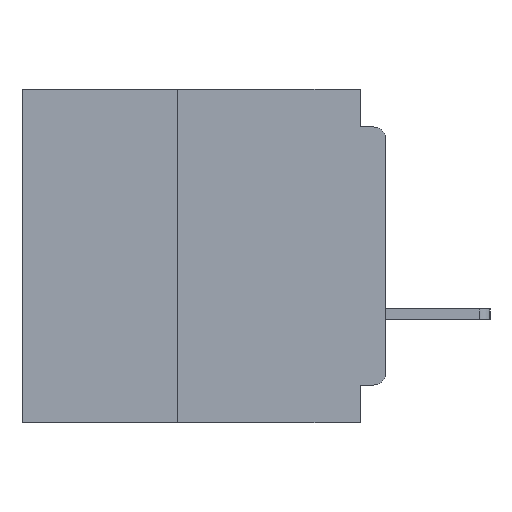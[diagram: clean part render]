
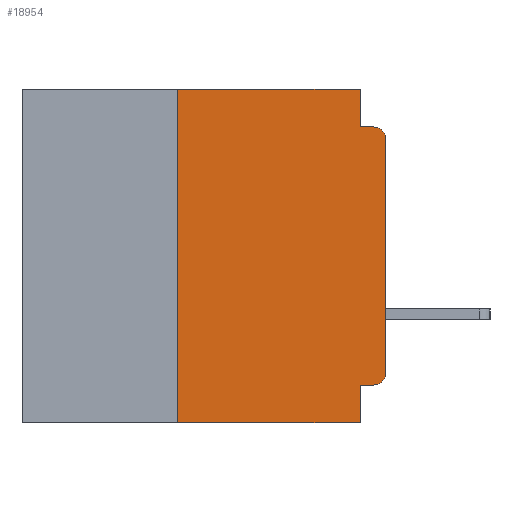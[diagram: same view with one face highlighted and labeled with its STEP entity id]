
A CAD part, left-side view. The second image highlights one B-rep face of the part: STEP entity #18954.
In plain terms, the highlighted planar face has unit normal (-1, 0, 0).
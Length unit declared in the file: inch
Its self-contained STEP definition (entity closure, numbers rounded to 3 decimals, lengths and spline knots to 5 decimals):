
#171 = EDGE_CURVE ( 'NONE', #24184, #37073, #20855, .T. ) ;
#1315 = EDGE_CURVE ( 'NONE', #27037, #25152, #16769, .T. ) ;
#1594 = VERTEX_POINT ( 'NONE', #29103 ) ;
#2092 = DIRECTION ( 'NONE',  ( 0., 0., -1. ) ) ;
#2588 = VECTOR ( 'NONE', #40106, 39.37008 ) ;
#3634 = PLANE ( 'NONE',  #33604 ) ;
#4364 = LINE ( 'NONE', #22673, #41997 ) ;
#5038 = ORIENTED_EDGE ( 'NONE', *, *, #36987, .T. ) ;
#8489 = VERTEX_POINT ( 'NONE', #29799 ) ;
#8672 = DIRECTION ( 'NONE',  ( 0., 1., 0. ) ) ;
#10243 = ORIENTED_EDGE ( 'NONE', *, *, #1315, .T. ) ;
#10694 = CARTESIAN_POINT ( 'NONE',  ( 0., 0.437, -0.4 ) ) ;
#10991 = DIRECTION ( 'NONE',  ( 1., 0., 0. ) ) ;
#11439 = CARTESIAN_POINT ( 'NONE',  ( 0., 0.031, -0.4 ) ) ;
#11780 = LINE ( 'NONE', #34227, #41982 ) ;
#11825 = DIRECTION ( 'NONE',  ( 0., -1., 0. ) ) ;
#12669 = EDGE_CURVE ( 'NONE', #1594, #23631, #24501, .T. ) ;
#12686 = ORIENTED_EDGE ( 'NONE', *, *, #22652, .F. ) ;
#12821 = CARTESIAN_POINT ( 'NONE',  ( 0., 0.25, -0.4 ) ) ;
#12879 = CARTESIAN_POINT ( 'NONE',  ( 0., 0.015, -0.045 ) ) ;
#13369 = DIRECTION ( 'NONE',  ( 0., 0., -1. ) ) ;
#13486 = CARTESIAN_POINT ( 'NONE',  ( 0., 0.015, -0.355 ) ) ;
#13913 = DIRECTION ( 'NONE',  ( -1., 0., 0. ) ) ;
#14073 = CARTESIAN_POINT ( 'NONE',  ( 0., 0.015, -0.34 ) ) ;
#14104 = EDGE_LOOP ( 'NONE', ( #5038, #17039, #27082, #12686, #37196, #30086, #36721, #33776, #36097, #10243 ) ) ;
#14174 = CARTESIAN_POINT ( 'NONE',  ( 0., 0., -0.045 ) ) ;
#14814 = CARTESIAN_POINT ( 'NONE',  ( 0., 0., -0.34 ) ) ;
#14836 = VECTOR ( 'NONE', #32329, 39.37008 ) ;
#15529 = CARTESIAN_POINT ( 'NONE',  ( 0., 0.015, -0.06 ) ) ;
#16284 = CARTESIAN_POINT ( 'NONE',  ( 0., 0., -0.06 ) ) ;
#16769 = CIRCLE ( 'NONE', #42944, 0.015 ) ;
#16864 = VERTEX_POINT ( 'NONE', #17652 ) ;
#17039 = ORIENTED_EDGE ( 'NONE', *, *, #42657, .T. ) ;
#17652 = CARTESIAN_POINT ( 'NONE',  ( 0., 0.25, 0. ) ) ;
#18551 = VECTOR ( 'NONE', #2092, 39.37008 ) ;
#18954 = ADVANCED_FACE ( 'NONE', ( #36962 ), #3634, .F. ) ;
#19143 = DIRECTION ( 'NONE',  ( 0., 0., -1. ) ) ;
#19571 = EDGE_CURVE ( 'NONE', #31402, #37073, #44894, .T. ) ;
#20855 = LINE ( 'NONE', #10694, #2588 ) ;
#21154 = EDGE_CURVE ( 'NONE', #16864, #8489, #4364, .T. ) ;
#21633 = CARTESIAN_POINT ( 'NONE',  ( 0., 0.031, -0.4 ) ) ;
#22652 = EDGE_CURVE ( 'NONE', #8489, #1594, #26007, .T. ) ;
#22673 = CARTESIAN_POINT ( 'NONE',  ( 0., 0.437, 0. ) ) ;
#23631 = VERTEX_POINT ( 'NONE', #12879 ) ;
#24184 = VERTEX_POINT ( 'NONE', #12821 ) ;
#24501 = LINE ( 'NONE', #14174, #14836 ) ;
#25152 = VERTEX_POINT ( 'NONE', #14814 ) ;
#25868 = CARTESIAN_POINT ( 'NONE',  ( 0., 0.25, -0.4 ) ) ;
#26007 = LINE ( 'NONE', #38465, #18551 ) ;
#27037 = VERTEX_POINT ( 'NONE', #13486 ) ;
#27082 = ORIENTED_EDGE ( 'NONE', *, *, #12669, .F. ) ;
#28520 = CARTESIAN_POINT ( 'NONE',  ( 0., 0., 0. ) ) ;
#28875 = EDGE_CURVE ( 'NONE', #24184, #16864, #33978, .T. ) ;
#29103 = CARTESIAN_POINT ( 'NONE',  ( 0., 0.031, -0.045 ) ) ;
#29539 = DIRECTION ( 'NONE',  ( 0., 0., 1. ) ) ;
#29777 = CIRCLE ( 'NONE', #32771, 0.015 ) ;
#29799 = CARTESIAN_POINT ( 'NONE',  ( 0., 0.031, 0. ) ) ;
#29803 = CARTESIAN_POINT ( 'NONE',  ( 0., 0.031, -0.355 ) ) ;
#30086 = ORIENTED_EDGE ( 'NONE', *, *, #28875, .F. ) ;
#31402 = VERTEX_POINT ( 'NONE', #29803 ) ;
#32329 = DIRECTION ( 'NONE',  ( 0., -1., 0. ) ) ;
#32771 = AXIS2_PLACEMENT_3D ( 'NONE', #15529, #40974, #19143 ) ;
#32841 = VECTOR ( 'NONE', #29539, 39.37008 ) ;
#32849 = CARTESIAN_POINT ( 'NONE',  ( 0., 0.437, 0. ) ) ;
#33604 = AXIS2_PLACEMENT_3D ( 'NONE', #32849, #10991, #36512 ) ;
#33776 = ORIENTED_EDGE ( 'NONE', *, *, #19571, .F. ) ;
#33978 = LINE ( 'NONE', #25868, #32841 ) ;
#34227 = CARTESIAN_POINT ( 'NONE',  ( 0., 0., -0.355 ) ) ;
#35179 = VECTOR ( 'NONE', #37110, 39.37008 ) ;
#35206 = VECTOR ( 'NONE', #43140, 39.37008 ) ;
#36097 = ORIENTED_EDGE ( 'NONE', *, *, #37322, .F. ) ;
#36512 = DIRECTION ( 'NONE',  ( 0., 0., -1. ) ) ;
#36721 = ORIENTED_EDGE ( 'NONE', *, *, #171, .T. ) ;
#36962 = FACE_OUTER_BOUND ( 'NONE', #14104, .T. ) ;
#36987 = EDGE_CURVE ( 'NONE', #25152, #42784, #44924, .T. ) ;
#37073 = VERTEX_POINT ( 'NONE', #21633 ) ;
#37110 = DIRECTION ( 'NONE',  ( 0., 0., -1. ) ) ;
#37196 = ORIENTED_EDGE ( 'NONE', *, *, #21154, .F. ) ;
#37322 = EDGE_CURVE ( 'NONE', #27037, #31402, #11780, .T. ) ;
#38465 = CARTESIAN_POINT ( 'NONE',  ( 0., 0.031, 0. ) ) ;
#40106 = DIRECTION ( 'NONE',  ( 0., -1., 0. ) ) ;
#40974 = DIRECTION ( 'NONE',  ( -1., 0., 0. ) ) ;
#41982 = VECTOR ( 'NONE', #8672, 39.37008 ) ;
#41997 = VECTOR ( 'NONE', #11825, 39.37008 ) ;
#42657 = EDGE_CURVE ( 'NONE', #42784, #23631, #29777, .T. ) ;
#42784 = VERTEX_POINT ( 'NONE', #16284 ) ;
#42944 = AXIS2_PLACEMENT_3D ( 'NONE', #14073, #13913, #13369 ) ;
#43140 = DIRECTION ( 'NONE',  ( 0., 0., 1. ) ) ;
#44894 = LINE ( 'NONE', #11439, #35179 ) ;
#44924 = LINE ( 'NONE', #28520, #35206 ) ;
